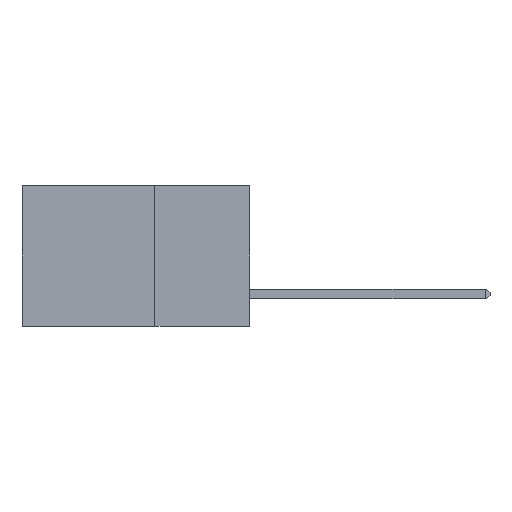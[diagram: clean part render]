
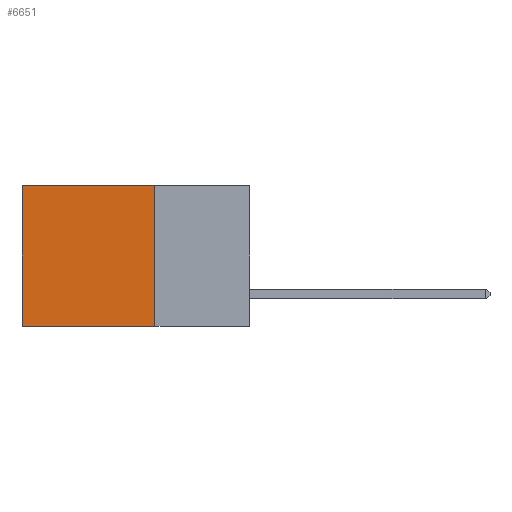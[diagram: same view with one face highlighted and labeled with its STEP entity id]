
A CAD part, left-side view. The second image highlights one B-rep face of the part: STEP entity #6651.
In plain terms, the highlighted planar face has unit normal (-1, 0, 0).
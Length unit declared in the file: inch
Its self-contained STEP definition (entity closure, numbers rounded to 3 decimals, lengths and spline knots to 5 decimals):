
#1360 = DIRECTION ( 'NONE',  ( 0., 0., -1. ) ) ;
#2082 = CARTESIAN_POINT ( 'NONE',  ( 0.2875, 0.25, -0.37 ) ) ;
#3624 = ORIENTED_EDGE ( 'NONE', *, *, #9304, .F. ) ;
#3659 = CARTESIAN_POINT ( 'NONE',  ( 0.2875, 0.25, 0. ) ) ;
#3675 = LINE ( 'NONE', #19456, #19234 ) ;
#5019 = EDGE_CURVE ( 'NONE', #23594, #27285, #30968, .T. ) ;
#5660 = ORIENTED_EDGE ( 'NONE', *, *, #5019, .T. ) ;
#6154 = VERTEX_POINT ( 'NONE', #2082 ) ;
#6645 = DIRECTION ( 'NONE',  ( 0., 0., -1. ) ) ;
#6651 = ADVANCED_FACE ( 'NONE', ( #26691 ), #29180, .F. ) ;
#8717 = EDGE_CURVE ( 'NONE', #6154, #16188, #3675, .T. ) ;
#9304 = EDGE_CURVE ( 'NONE', #23594, #6154, #13903, .T. ) ;
#12492 = CARTESIAN_POINT ( 'NONE',  ( 0.2875, 0.6, 0. ) ) ;
#13158 = EDGE_CURVE ( 'NONE', #27285, #16188, #17509, .T. ) ;
#13712 = CARTESIAN_POINT ( 'NONE',  ( 0.2875, 0.25, 0. ) ) ;
#13903 = LINE ( 'NONE', #3659, #21197 ) ;
#14461 = VECTOR ( 'NONE', #36412, 39.37008 ) ;
#16188 = VERTEX_POINT ( 'NONE', #29714 ) ;
#16524 = CARTESIAN_POINT ( 'NONE',  ( 0.2875, 0.6, 0. ) ) ;
#17509 = LINE ( 'NONE', #12492, #18505 ) ;
#18505 = VECTOR ( 'NONE', #34228, 39.37008 ) ;
#18980 = AXIS2_PLACEMENT_3D ( 'NONE', #13712, #19969, #1360 ) ;
#19234 = VECTOR ( 'NONE', #38077, 39.37008 ) ;
#19456 = CARTESIAN_POINT ( 'NONE',  ( 0.2875, 0.25, -0.37 ) ) ;
#19969 = DIRECTION ( 'NONE',  ( 1., 0., 0. ) ) ;
#21197 = VECTOR ( 'NONE', #6645, 39.37008 ) ;
#23253 = ORIENTED_EDGE ( 'NONE', *, *, #8717, .F. ) ;
#23594 = VERTEX_POINT ( 'NONE', #31528 ) ;
#25477 = EDGE_LOOP ( 'NONE', ( #29139, #23253, #3624, #5660 ) ) ;
#26691 = FACE_OUTER_BOUND ( 'NONE', #25477, .T. ) ;
#27285 = VERTEX_POINT ( 'NONE', #16524 ) ;
#29139 = ORIENTED_EDGE ( 'NONE', *, *, #13158, .T. ) ;
#29180 = PLANE ( 'NONE',  #18980 ) ;
#29714 = CARTESIAN_POINT ( 'NONE',  ( 0.2875, 0.6, -0.37 ) ) ;
#30103 = CARTESIAN_POINT ( 'NONE',  ( 0.2875, 0.25, 0. ) ) ;
#30968 = LINE ( 'NONE', #30103, #14461 ) ;
#31528 = CARTESIAN_POINT ( 'NONE',  ( 0.2875, 0.25, 0. ) ) ;
#34228 = DIRECTION ( 'NONE',  ( 0., 0., -1. ) ) ;
#36412 = DIRECTION ( 'NONE',  ( 0., 1., 0. ) ) ;
#38077 = DIRECTION ( 'NONE',  ( 0., 1., 0. ) ) ;
